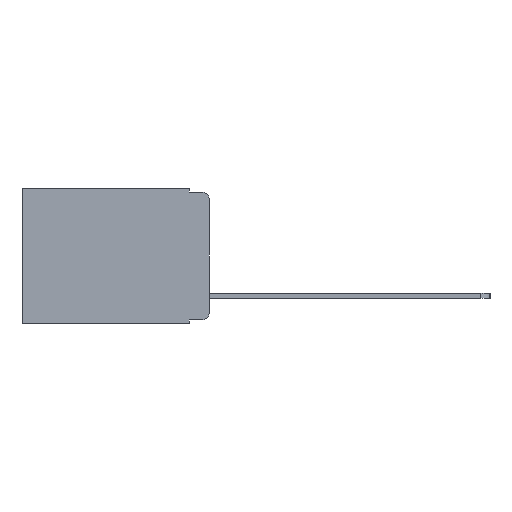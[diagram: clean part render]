
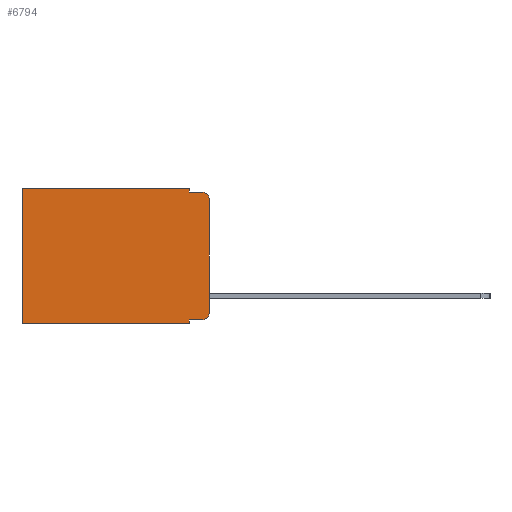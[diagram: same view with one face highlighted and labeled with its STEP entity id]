
A CAD part, left-side view. The second image highlights one B-rep face of the part: STEP entity #6794.
In plain terms, the highlighted planar face has unit normal (-1, 0, 0).
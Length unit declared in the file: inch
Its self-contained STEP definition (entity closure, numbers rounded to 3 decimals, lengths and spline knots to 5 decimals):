
#156 = EDGE_CURVE ( 'NONE', #6069, #9695, #13204, .T. ) ;
#385 = PLANE ( 'NONE',  #7457 ) ;
#632 = CARTESIAN_POINT ( 'NONE',  ( 0.298, 0.051, 0. ) ) ;
#955 = CARTESIAN_POINT ( 'NONE',  ( 0.298, 0.473, 0. ) ) ;
#1066 = VECTOR ( 'NONE', #12513, 39.37008 ) ;
#1147 = CARTESIAN_POINT ( 'NONE',  ( 0.298, 0., -0.03 ) ) ;
#1252 = CARTESIAN_POINT ( 'NONE',  ( 0.298, 0., 0. ) ) ;
#1458 = AXIS2_PLACEMENT_3D ( 'NONE', #1574, #2755, #2723 ) ;
#1481 = AXIS2_PLACEMENT_3D ( 'NONE', #2112, #10266, #3349 ) ;
#1574 = CARTESIAN_POINT ( 'NONE',  ( 0.298, 0.02, -0.03 ) ) ;
#2112 = CARTESIAN_POINT ( 'NONE',  ( 0.298, 0.02, -0.313 ) ) ;
#2654 = LINE ( 'NONE', #9318, #11441 ) ;
#2685 = VERTEX_POINT ( 'NONE', #13096 ) ;
#2709 = CARTESIAN_POINT ( 'NONE',  ( 0.298, 0., 0. ) ) ;
#2723 = DIRECTION ( 'NONE',  ( 0., 0., -1. ) ) ;
#2755 = DIRECTION ( 'NONE',  ( -1., 0., 0. ) ) ;
#2984 = DIRECTION ( 'NONE',  ( 1., 0., 0. ) ) ;
#3087 = ORIENTED_EDGE ( 'NONE', *, *, #6415, .T. ) ;
#3174 = EDGE_CURVE ( 'NONE', #6975, #11520, #10693, .T. ) ;
#3260 = CARTESIAN_POINT ( 'NONE',  ( 0.298, 0.051, 0. ) ) ;
#3349 = DIRECTION ( 'NONE',  ( 0., 0., -1. ) ) ;
#3411 = ORIENTED_EDGE ( 'NONE', *, *, #14233, .F. ) ;
#3426 = ORIENTED_EDGE ( 'NONE', *, *, #13880, .F. ) ;
#3481 = DIRECTION ( 'NONE',  ( 0., 1., 0. ) ) ;
#3656 = ORIENTED_EDGE ( 'NONE', *, *, #156, .T. ) ;
#3864 = VECTOR ( 'NONE', #14605, 39.37008 ) ;
#3945 = DIRECTION ( 'NONE',  ( 0., 0., -1. ) ) ;
#4334 = ORIENTED_EDGE ( 'NONE', *, *, #10703, .F. ) ;
#4397 = ORIENTED_EDGE ( 'NONE', *, *, #3174, .T. ) ;
#4708 = CARTESIAN_POINT ( 'NONE',  ( 0.298, 0.473, -0.343 ) ) ;
#4834 = VERTEX_POINT ( 'NONE', #6070 ) ;
#4944 = LINE ( 'NONE', #12450, #8062 ) ;
#5459 = EDGE_CURVE ( 'NONE', #12904, #2685, #2654, .T. ) ;
#5775 = VECTOR ( 'NONE', #10154, 39.37008 ) ;
#6004 = CARTESIAN_POINT ( 'NONE',  ( 0.298, 0.051, 0. ) ) ;
#6069 = VERTEX_POINT ( 'NONE', #1147 ) ;
#6070 = CARTESIAN_POINT ( 'NONE',  ( 0.298, 0., -0.313 ) ) ;
#6361 = LINE ( 'NONE', #955, #12522 ) ;
#6415 = EDGE_CURVE ( 'NONE', #11520, #14042, #6361, .T. ) ;
#6754 = ORIENTED_EDGE ( 'NONE', *, *, #5459, .T. ) ;
#6794 = ADVANCED_FACE ( 'NONE', ( #10424 ), #385, .F. ) ;
#6812 = ORIENTED_EDGE ( 'NONE', *, *, #13130, .T. ) ;
#6975 = VERTEX_POINT ( 'NONE', #3260 ) ;
#7104 = ORIENTED_EDGE ( 'NONE', *, *, #9827, .F. ) ;
#7145 = ORIENTED_EDGE ( 'NONE', *, *, #11471, .F. ) ;
#7254 = CARTESIAN_POINT ( 'NONE',  ( 0.298, 0.473, 0. ) ) ;
#7387 = VERTEX_POINT ( 'NONE', #11961 ) ;
#7417 = CARTESIAN_POINT ( 'NONE',  ( 0.298, 0.051, -0.343 ) ) ;
#7457 = AXIS2_PLACEMENT_3D ( 'NONE', #8835, #2984, #11029 ) ;
#7893 = VECTOR ( 'NONE', #13704, 39.37008 ) ;
#8062 = VECTOR ( 'NONE', #3481, 39.37008 ) ;
#8097 = VERTEX_POINT ( 'NONE', #7417 ) ;
#8108 = EDGE_LOOP ( 'NONE', ( #3411, #3656, #4334, #3426, #4397, #3087, #7104, #7145, #6754, #6812 ) ) ;
#8180 = DIRECTION ( 'NONE',  ( 0., -1., 0. ) ) ;
#8835 = CARTESIAN_POINT ( 'NONE',  ( 0.298, 0., 0. ) ) ;
#9192 = VECTOR ( 'NONE', #3945, 39.37008 ) ;
#9286 = DIRECTION ( 'NONE',  ( 0., 0., -1. ) ) ;
#9318 = CARTESIAN_POINT ( 'NONE',  ( 0.298, 0.051, -0.333 ) ) ;
#9570 = LINE ( 'NONE', #2709, #9192 ) ;
#9695 = VERTEX_POINT ( 'NONE', #11863 ) ;
#9827 = EDGE_CURVE ( 'NONE', #8097, #14042, #4944, .T. ) ;
#10154 = DIRECTION ( 'NONE',  ( 0., 0., -1. ) ) ;
#10266 = DIRECTION ( 'NONE',  ( -1., 0., 0. ) ) ;
#10424 = FACE_OUTER_BOUND ( 'NONE', #8108, .T. ) ;
#10693 = LINE ( 'NONE', #1252, #3864 ) ;
#10703 = EDGE_CURVE ( 'NONE', #7387, #9695, #13221, .T. ) ;
#10846 = LINE ( 'NONE', #6004, #7893 ) ;
#11029 = DIRECTION ( 'NONE',  ( 0., 0., -1. ) ) ;
#11441 = VECTOR ( 'NONE', #8180, 39.37008 ) ;
#11471 = EDGE_CURVE ( 'NONE', #12904, #8097, #10846, .T. ) ;
#11498 = CARTESIAN_POINT ( 'NONE',  ( 0.298, 0.051, -0.01 ) ) ;
#11520 = VERTEX_POINT ( 'NONE', #7254 ) ;
#11863 = CARTESIAN_POINT ( 'NONE',  ( 0.298, 0.02, -0.01 ) ) ;
#11961 = CARTESIAN_POINT ( 'NONE',  ( 0.298, 0.051, -0.01 ) ) ;
#12038 = LINE ( 'NONE', #632, #5775 ) ;
#12450 = CARTESIAN_POINT ( 'NONE',  ( 0.298, 0., -0.343 ) ) ;
#12513 = DIRECTION ( 'NONE',  ( 0., -1., 0. ) ) ;
#12522 = VECTOR ( 'NONE', #9286, 39.37008 ) ;
#12904 = VERTEX_POINT ( 'NONE', #13990 ) ;
#13096 = CARTESIAN_POINT ( 'NONE',  ( 0.298, 0.02, -0.333 ) ) ;
#13130 = EDGE_CURVE ( 'NONE', #2685, #4834, #14599, .T. ) ;
#13204 = CIRCLE ( 'NONE', #1458, 0.02 ) ;
#13221 = LINE ( 'NONE', #11498, #1066 ) ;
#13704 = DIRECTION ( 'NONE',  ( 0., 0., -1. ) ) ;
#13880 = EDGE_CURVE ( 'NONE', #6975, #7387, #12038, .T. ) ;
#13990 = CARTESIAN_POINT ( 'NONE',  ( 0.298, 0.051, -0.333 ) ) ;
#14042 = VERTEX_POINT ( 'NONE', #4708 ) ;
#14233 = EDGE_CURVE ( 'NONE', #6069, #4834, #9570, .T. ) ;
#14599 = CIRCLE ( 'NONE', #1481, 0.02 ) ;
#14605 = DIRECTION ( 'NONE',  ( 0., 1., 0. ) ) ;
